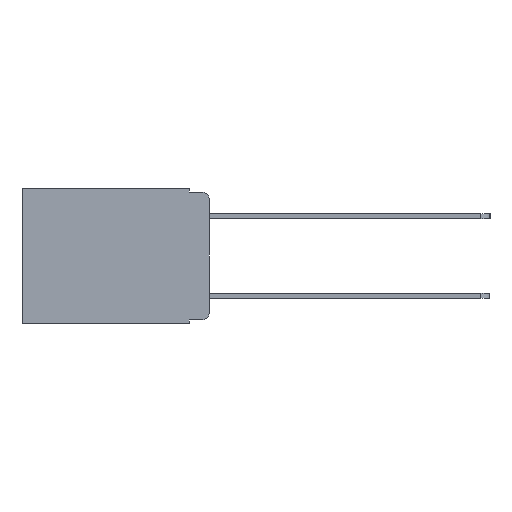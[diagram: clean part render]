
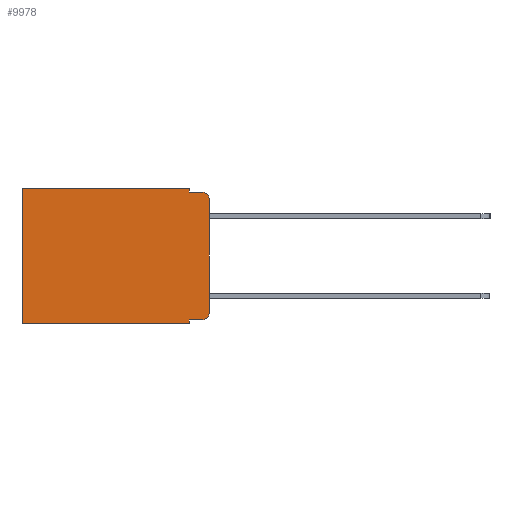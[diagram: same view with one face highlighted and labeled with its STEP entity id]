
A CAD part, left-side view. The second image highlights one B-rep face of the part: STEP entity #9978.
In plain terms, the highlighted planar face has unit normal (-1, 0, 0).
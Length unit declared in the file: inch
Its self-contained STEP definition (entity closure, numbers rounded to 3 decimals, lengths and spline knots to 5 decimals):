
#168 = VECTOR ( 'NONE', #16312, 39.37008 ) ;
#240 = VECTOR ( 'NONE', #9414, 39.37008 ) ;
#510 = DIRECTION ( 'NONE',  ( 0., 0., -1. ) ) ;
#558 = CARTESIAN_POINT ( 'NONE',  ( 0.298, 0., -0.313 ) ) ;
#608 = VERTEX_POINT ( 'NONE', #18376 ) ;
#686 = LINE ( 'NONE', #1483, #168 ) ;
#1357 = VERTEX_POINT ( 'NONE', #6049 ) ;
#1483 = CARTESIAN_POINT ( 'NONE',  ( 0.298, 0.051, 0. ) ) ;
#1613 = ORIENTED_EDGE ( 'NONE', *, *, #8244, .F. ) ;
#1678 = EDGE_LOOP ( 'NONE', ( #10205, #10507, #1613, #20977, #10335, #19273, #6434, #14756, #7954, #17724 ) ) ;
#1911 = DIRECTION ( 'NONE',  ( 0., 0., -1. ) ) ;
#1936 = VERTEX_POINT ( 'NONE', #2715 ) ;
#2715 = CARTESIAN_POINT ( 'NONE',  ( 0.298, 0.051, -0.01 ) ) ;
#2890 = CARTESIAN_POINT ( 'NONE',  ( 0.298, 0.02, -0.01 ) ) ;
#3044 = VECTOR ( 'NONE', #20388, 39.37008 ) ;
#3654 = CARTESIAN_POINT ( 'NONE',  ( 0.298, 0., 0. ) ) ;
#4042 = VERTEX_POINT ( 'NONE', #4103 ) ;
#4061 = CARTESIAN_POINT ( 'NONE',  ( 0.298, 0.051, -0.333 ) ) ;
#4103 = CARTESIAN_POINT ( 'NONE',  ( 0.298, 0.051, 0. ) ) ;
#4160 = DIRECTION ( 'NONE',  ( 0., -1., 0. ) ) ;
#4391 = VECTOR ( 'NONE', #510, 39.37008 ) ;
#4410 = LINE ( 'NONE', #4061, #20876 ) ;
#4731 = VERTEX_POINT ( 'NONE', #11066 ) ;
#5782 = AXIS2_PLACEMENT_3D ( 'NONE', #3654, #8780, #20238 ) ;
#5904 = EDGE_CURVE ( 'NONE', #1357, #15088, #4410, .T. ) ;
#6037 = DIRECTION ( 'NONE',  ( 0., 0., -1. ) ) ;
#6049 = CARTESIAN_POINT ( 'NONE',  ( 0.298, 0.051, -0.333 ) ) ;
#6263 = EDGE_CURVE ( 'NONE', #9415, #13439, #18047, .T. ) ;
#6434 = ORIENTED_EDGE ( 'NONE', *, *, #10929, .F. ) ;
#6507 = EDGE_CURVE ( 'NONE', #4042, #20008, #9087, .T. ) ;
#7090 = PLANE ( 'NONE',  #5782 ) ;
#7243 = CARTESIAN_POINT ( 'NONE',  ( 0.298, 0.051, -0.01 ) ) ;
#7683 = VECTOR ( 'NONE', #6037, 39.37008 ) ;
#7753 = EDGE_CURVE ( 'NONE', #15088, #13439, #12147, .T. ) ;
#7954 = ORIENTED_EDGE ( 'NONE', *, *, #5904, .T. ) ;
#8136 = CARTESIAN_POINT ( 'NONE',  ( 0.298, 0., -0.343 ) ) ;
#8244 = EDGE_CURVE ( 'NONE', #1936, #21133, #20590, .T. ) ;
#8780 = DIRECTION ( 'NONE',  ( 1., 0., 0. ) ) ;
#8798 = CARTESIAN_POINT ( 'NONE',  ( 0.298, 0., 0. ) ) ;
#9087 = LINE ( 'NONE', #11019, #240 ) ;
#9351 = DIRECTION ( 'NONE',  ( -1., 0., 0. ) ) ;
#9370 = DIRECTION ( 'NONE',  ( -1., 0., 0. ) ) ;
#9414 = DIRECTION ( 'NONE',  ( 0., 1., 0. ) ) ;
#9415 = VERTEX_POINT ( 'NONE', #10628 ) ;
#9978 = ADVANCED_FACE ( 'NONE', ( #17681 ), #7090, .F. ) ;
#10205 = ORIENTED_EDGE ( 'NONE', *, *, #6263, .F. ) ;
#10335 = ORIENTED_EDGE ( 'NONE', *, *, #6507, .T. ) ;
#10459 = CIRCLE ( 'NONE', #11635, 0.02 ) ;
#10507 = ORIENTED_EDGE ( 'NONE', *, *, #20074, .T. ) ;
#10628 = CARTESIAN_POINT ( 'NONE',  ( 0.298, 0., -0.03 ) ) ;
#10929 = EDGE_CURVE ( 'NONE', #4731, #608, #12794, .T. ) ;
#11019 = CARTESIAN_POINT ( 'NONE',  ( 0.298, 0., 0. ) ) ;
#11066 = CARTESIAN_POINT ( 'NONE',  ( 0.298, 0.051, -0.343 ) ) ;
#11635 = AXIS2_PLACEMENT_3D ( 'NONE', #19152, #9351, #20805 ) ;
#11900 = CARTESIAN_POINT ( 'NONE',  ( 0.298, 0.02, -0.333 ) ) ;
#12147 = CIRCLE ( 'NONE', #12445, 0.02 ) ;
#12445 = AXIS2_PLACEMENT_3D ( 'NONE', #19170, #9370, #20823 ) ;
#12794 = LINE ( 'NONE', #8136, #20465 ) ;
#13439 = VERTEX_POINT ( 'NONE', #558 ) ;
#14756 = ORIENTED_EDGE ( 'NONE', *, *, #15708, .F. ) ;
#15088 = VERTEX_POINT ( 'NONE', #11900 ) ;
#15708 = EDGE_CURVE ( 'NONE', #1357, #4731, #20635, .T. ) ;
#15747 = CARTESIAN_POINT ( 'NONE',  ( 0.298, 0.473, 0. ) ) ;
#16312 = DIRECTION ( 'NONE',  ( 0., 0., -1. ) ) ;
#16727 = CARTESIAN_POINT ( 'NONE',  ( 0.298, 0.051, 0. ) ) ;
#16956 = LINE ( 'NONE', #20853, #7683 ) ;
#17681 = FACE_OUTER_BOUND ( 'NONE', #1678, .T. ) ;
#17724 = ORIENTED_EDGE ( 'NONE', *, *, #7753, .T. ) ;
#17799 = EDGE_CURVE ( 'NONE', #4042, #1936, #686, .T. ) ;
#18047 = LINE ( 'NONE', #8798, #4391 ) ;
#18376 = CARTESIAN_POINT ( 'NONE',  ( 0.298, 0.473, -0.343 ) ) ;
#18812 = EDGE_CURVE ( 'NONE', #20008, #608, #16956, .T. ) ;
#19152 = CARTESIAN_POINT ( 'NONE',  ( 0.298, 0.02, -0.03 ) ) ;
#19170 = CARTESIAN_POINT ( 'NONE',  ( 0.298, 0.02, -0.313 ) ) ;
#19273 = ORIENTED_EDGE ( 'NONE', *, *, #18812, .T. ) ;
#20008 = VERTEX_POINT ( 'NONE', #15747 ) ;
#20074 = EDGE_CURVE ( 'NONE', #9415, #21133, #10459, .T. ) ;
#20128 = VECTOR ( 'NONE', #1911, 39.37008 ) ;
#20238 = DIRECTION ( 'NONE',  ( 0., 0., -1. ) ) ;
#20388 = DIRECTION ( 'NONE',  ( 0., -1., 0. ) ) ;
#20465 = VECTOR ( 'NONE', #21227, 39.37008 ) ;
#20590 = LINE ( 'NONE', #7243, #3044 ) ;
#20635 = LINE ( 'NONE', #16727, #20128 ) ;
#20805 = DIRECTION ( 'NONE',  ( 0., 0., -1. ) ) ;
#20823 = DIRECTION ( 'NONE',  ( 0., 0., -1. ) ) ;
#20853 = CARTESIAN_POINT ( 'NONE',  ( 0.298, 0.473, 0. ) ) ;
#20876 = VECTOR ( 'NONE', #4160, 39.37008 ) ;
#20977 = ORIENTED_EDGE ( 'NONE', *, *, #17799, .F. ) ;
#21133 = VERTEX_POINT ( 'NONE', #2890 ) ;
#21227 = DIRECTION ( 'NONE',  ( 0., 1., 0. ) ) ;
